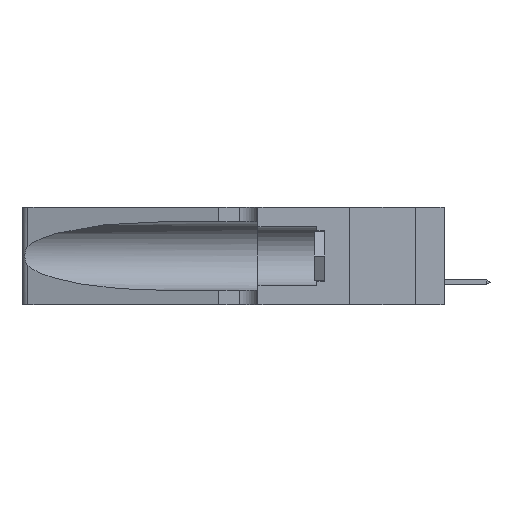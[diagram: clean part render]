
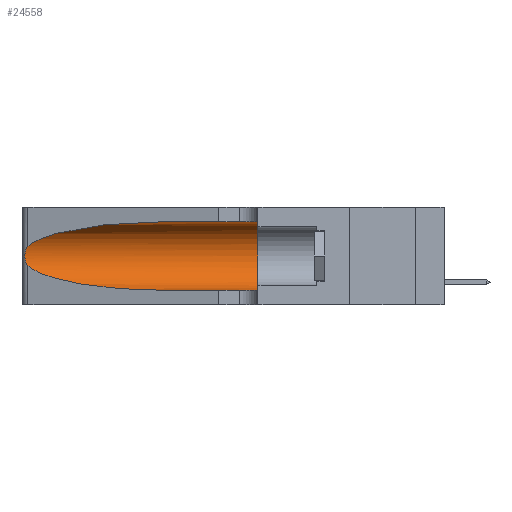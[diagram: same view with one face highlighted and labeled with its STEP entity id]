
A CAD part, left-side view. The second image highlights one B-rep face of the part: STEP entity #24558.
In plain terms, the highlighted cylindrical face has radius 3.308 mm (diameter 6.617 mm), a partial arc.
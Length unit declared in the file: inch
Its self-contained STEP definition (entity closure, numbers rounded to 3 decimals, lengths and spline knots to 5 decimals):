
#830 = CARTESIAN_POINT ( 'NONE',  ( 0.26017, 1.23833, 0.17102 ) ) ;
#1282 = CARTESIAN_POINT ( 'NONE',  ( 0.18966, 0.96281, 0.05475 ) ) ;
#1574 = ORIENTED_EDGE ( 'NONE', *, *, #28122, .T. ) ;
#1807 = LINE ( 'NONE', #9940, #14302 ) ;
#2654 = CARTESIAN_POINT ( 'NONE',  ( 0.25487, 1.22718, 0.22369 ) ) ;
#2684 = CARTESIAN_POINT ( 'NONE',  ( 0.1305, 0.72297, 0.31525 ) ) ;
#3043 = CARTESIAN_POINT ( 'NONE',  ( 0.25639, 1.23184, 0.21858 ) ) ;
#3171 = VERTEX_POINT ( 'NONE', #2654 ) ;
#3336 = CARTESIAN_POINT ( 'NONE',  ( 0.25487, 1.22718, 0.14631 ) ) ;
#3384 = CARTESIAN_POINT ( 'NONE',  ( 0.2373, 1.15595, 0.08982 ) ) ;
#3443 = EDGE_LOOP ( 'NONE', ( #24372, #1574, #9719, #25222, #13346, #23017 ) ) ;
#4505 = LINE ( 'NONE', #24090, #28157 ) ;
#5192 = EDGE_CURVE ( 'NONE', #20480, #19340, #1807, .T. ) ;
#6453 = CYLINDRICAL_SURFACE ( 'NONE', #16585, 0.13025 ) ;
#6495 = VERTEX_POINT ( 'NONE', #13832 ) ;
#7353 = CARTESIAN_POINT ( 'NONE',  ( 0.25487, 1.22718, 0.22369 ) ) ;
#7524 = CARTESIAN_POINT ( 'NONE',  ( 0.1305, 0.35, 0.31525 ) ) ;
#7906 = CARTESIAN_POINT ( 'NONE',  ( 0.25787, 1.23484, 0.2124 ) ) ;
#8798 = EDGE_CURVE ( 'NONE', #21358, #14800, #10531, .T. ) ;
#9142 = CARTESIAN_POINT ( 'NONE',  ( 0.1305, 0.72297, 0.05475 ) ) ;
#9212 = B_SPLINE_CURVE_WITH_KNOTS ( 'NONE', 3,
 ( #26073, #26267, #3043, #7906, #21532, #12199, #17017, #28362, #830, #28265, #14502, #12308, #12504, #3336 ),
 .UNSPECIFIED., .F., .F.,
 ( 4, 2, 2, 2, 2, 2, 4 ),
 ( 0., 0.00027, 0.00053, 0.00107, 0.0016, 0.00187, 0.00214 ),
 .UNSPECIFIED. ) ;
#9719 = ORIENTED_EDGE ( 'NONE', *, *, #8798, .T. ) ;
#9940 = CARTESIAN_POINT ( 'NONE',  ( 0.1305, 1.61858, 0.31525 ) ) ;
#10531 =( BOUNDED_CURVE ( )  B_SPLINE_CURVE ( 3, ( #28603, #3384, #1282, #19255 ),
 .UNSPECIFIED., .F., .F. ) 
 B_SPLINE_CURVE_WITH_KNOTS ( ( 4, 4 ),
 ( 3.44316, 4.71239 ),
 .UNSPECIFIED. ) 
 CURVE ( )  GEOMETRIC_REPRESENTATION_ITEM ( )  RATIONAL_B_SPLINE_CURVE ( ( 1., 0.87, 0.87, 1. ) ) 
 REPRESENTATION_ITEM ( '' )  );
#10562 = CARTESIAN_POINT ( 'NONE',  ( 0.1305, 0.35, 0.185 ) ) ;
#12199 = CARTESIAN_POINT ( 'NONE',  ( 0.26018, 1.23835, 0.19895 ) ) ;
#12308 = CARTESIAN_POINT ( 'NONE',  ( 0.25639, 1.23186, 0.15144 ) ) ;
#12427 = DIRECTION ( 'NONE',  ( 0., -1., 0. ) ) ;
#12504 = CARTESIAN_POINT ( 'NONE',  ( 0.25555, 1.22993, 0.14849 ) ) ;
#12521 = CARTESIAN_POINT ( 'NONE',  ( 0.25487, 1.22718, 0.14631 ) ) ;
#13346 = ORIENTED_EDGE ( 'NONE', *, *, #29495, .F. ) ;
#13832 = CARTESIAN_POINT ( 'NONE',  ( 0.1305, 0.35, 0.05475 ) ) ;
#13991 = CARTESIAN_POINT ( 'NONE',  ( 0.1305, 1.61858, 0.185 ) ) ;
#14302 = VECTOR ( 'NONE', #12427, 39.37008 ) ;
#14502 = CARTESIAN_POINT ( 'NONE',  ( 0.25789, 1.23486, 0.15765 ) ) ;
#14800 = VERTEX_POINT ( 'NONE', #9142 ) ;
#16561 = CARTESIAN_POINT ( 'NONE',  ( 0.2373, 1.15595, 0.28018 ) ) ;
#16585 = AXIS2_PLACEMENT_3D ( 'NONE', #13991, #20884, #22518 ) ;
#16748 = CARTESIAN_POINT ( 'NONE',  ( 0.18966, 0.96281, 0.31525 ) ) ;
#17017 = CARTESIAN_POINT ( 'NONE',  ( 0.26075, 1.23896, 0.19203 ) ) ;
#18661 = CARTESIAN_POINT ( 'NONE',  ( 0.1305, 0.72297, 0.31525 ) ) ;
#19255 = CARTESIAN_POINT ( 'NONE',  ( 0.1305, 0.72297, 0.05475 ) ) ;
#19340 = VERTEX_POINT ( 'NONE', #7524 ) ;
#20480 = VERTEX_POINT ( 'NONE', #2684 ) ;
#20588 = CIRCLE ( 'NONE', #28386, 0.13025 ) ;
#20712 = EDGE_CURVE ( 'NONE', #14800, #6495, #4505, .T. ) ;
#20884 = DIRECTION ( 'NONE',  ( 0., -1., 0. ) ) ;
#21358 = VERTEX_POINT ( 'NONE', #12521 ) ;
#21532 = CARTESIAN_POINT ( 'NONE',  ( 0.25854, 1.2359, 0.20912 ) ) ;
#22518 = DIRECTION ( 'NONE',  ( 0., 0., -1. ) ) ;
#23017 = ORIENTED_EDGE ( 'NONE', *, *, #5192, .F. ) ;
#23437 = EDGE_CURVE ( 'NONE', #20480, #3171, #27807, .T. ) ;
#24090 = CARTESIAN_POINT ( 'NONE',  ( 0.1305, 1.61858, 0.05475 ) ) ;
#24372 = ORIENTED_EDGE ( 'NONE', *, *, #23437, .T. ) ;
#24558 = ADVANCED_FACE ( 'NONE', ( #28309 ), #6453, .F. ) ;
#25222 = ORIENTED_EDGE ( 'NONE', *, *, #20712, .T. ) ;
#26073 = CARTESIAN_POINT ( 'NONE',  ( 0.25487, 1.22718, 0.22369 ) ) ;
#26267 = CARTESIAN_POINT ( 'NONE',  ( 0.25555, 1.22994, 0.2215 ) ) ;
#26697 = DIRECTION ( 'NONE',  ( 0., 1., 0. ) ) ;
#27807 =( BOUNDED_CURVE ( )  B_SPLINE_CURVE ( 3, ( #18661, #16748, #16561, #7353 ),
 .UNSPECIFIED., .F., .T. ) 
 B_SPLINE_CURVE_WITH_KNOTS ( ( 4, 4 ),
 ( 1.5708, 2.84003 ),
 .UNSPECIFIED. ) 
 CURVE ( )  GEOMETRIC_REPRESENTATION_ITEM ( )  RATIONAL_B_SPLINE_CURVE ( ( 1., 0.87, 0.87, 1. ) ) 
 REPRESENTATION_ITEM ( '' )  );
#28122 = EDGE_CURVE ( 'NONE', #3171, #21358, #9212, .T. ) ;
#28157 = VECTOR ( 'NONE', #28912, 39.37008 ) ;
#28265 = CARTESIAN_POINT ( 'NONE',  ( 0.25856, 1.23593, 0.16098 ) ) ;
#28309 = FACE_OUTER_BOUND ( 'NONE', #3443, .T. ) ;
#28362 = CARTESIAN_POINT ( 'NONE',  ( 0.26075, 1.23896, 0.178 ) ) ;
#28386 = AXIS2_PLACEMENT_3D ( 'NONE', #10562, #26697, #28902 ) ;
#28603 = CARTESIAN_POINT ( 'NONE',  ( 0.25487, 1.22718, 0.14631 ) ) ;
#28902 = DIRECTION ( 'NONE',  ( 0., 0., 1. ) ) ;
#28912 = DIRECTION ( 'NONE',  ( 0., -1., 0. ) ) ;
#29495 = EDGE_CURVE ( 'NONE', #19340, #6495, #20588, .T. ) ;
